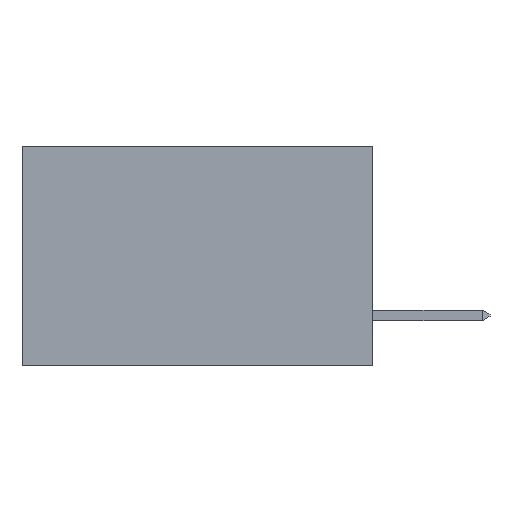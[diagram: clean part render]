
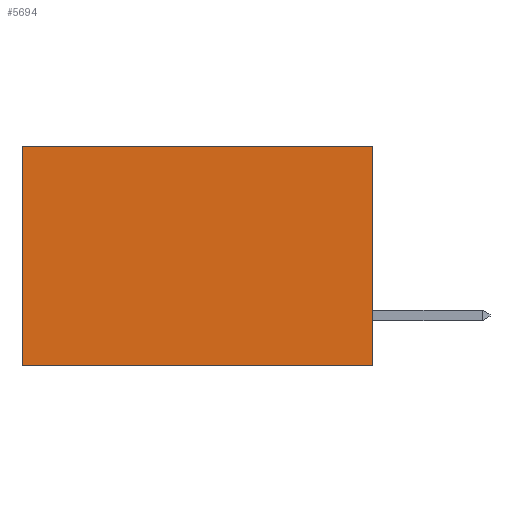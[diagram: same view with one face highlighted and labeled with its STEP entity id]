
A CAD part, left-side view. The second image highlights one B-rep face of the part: STEP entity #5694.
In plain terms, the highlighted planar face has unit normal (-1, 0, 0).
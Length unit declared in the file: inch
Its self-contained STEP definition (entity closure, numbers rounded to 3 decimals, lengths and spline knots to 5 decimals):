
#236 = AXIS2_PLACEMENT_3D ( 'NONE', #5465, #4556, #4618 ) ;
#449 = LINE ( 'NONE', #5411, #7240 ) ;
#672 = VERTEX_POINT ( 'NONE', #8423 ) ;
#1122 = DIRECTION ( 'NONE',  ( 0., 1., 0. ) ) ;
#1736 = EDGE_LOOP ( 'NONE', ( #2048, #1748, #2579, #3522 ) ) ;
#1748 = ORIENTED_EDGE ( 'NONE', *, *, #2026, .F. ) ;
#1870 = LINE ( 'NONE', #3115, #6932 ) ;
#2026 = EDGE_CURVE ( 'NONE', #7557, #6069, #7867, .T. ) ;
#2048 = ORIENTED_EDGE ( 'NONE', *, *, #3025, .T. ) ;
#2579 = ORIENTED_EDGE ( 'NONE', *, *, #5147, .F. ) ;
#2893 = PLANE ( 'NONE',  #236 ) ;
#3025 = EDGE_CURVE ( 'NONE', #672, #6069, #449, .T. ) ;
#3115 = CARTESIAN_POINT ( 'NONE',  ( 0.277, 0., 0. ) ) ;
#3223 = EDGE_CURVE ( 'NONE', #8510, #672, #1870, .T. ) ;
#3522 = ORIENTED_EDGE ( 'NONE', *, *, #3223, .T. ) ;
#4412 = VECTOR ( 'NONE', #7350, 39.37008 ) ;
#4425 = VECTOR ( 'NONE', #6179, 39.37008 ) ;
#4556 = DIRECTION ( 'NONE',  ( 1., 0., 0. ) ) ;
#4618 = DIRECTION ( 'NONE',  ( 0., 0., -1. ) ) ;
#4619 = LINE ( 'NONE', #7349, #4412 ) ;
#4814 = CARTESIAN_POINT ( 'NONE',  ( 0.277, 0., -0.37 ) ) ;
#5106 = FACE_OUTER_BOUND ( 'NONE', #1736, .T. ) ;
#5129 = DIRECTION ( 'NONE',  ( 0., 0., -1. ) ) ;
#5147 = EDGE_CURVE ( 'NONE', #8510, #7557, #4619, .T. ) ;
#5411 = CARTESIAN_POINT ( 'NONE',  ( 0.277, 0.59, -0.37 ) ) ;
#5465 = CARTESIAN_POINT ( 'NONE',  ( 0.277, 0., -0.37 ) ) ;
#5597 = CARTESIAN_POINT ( 'NONE',  ( 0.277, 0., 0. ) ) ;
#5694 = ADVANCED_FACE ( 'NONE', ( #5106 ), #2893, .F. ) ;
#6069 = VERTEX_POINT ( 'NONE', #8297 ) ;
#6074 = CARTESIAN_POINT ( 'NONE',  ( 0.277, 0., -0.37 ) ) ;
#6179 = DIRECTION ( 'NONE',  ( 0., 1., 0. ) ) ;
#6932 = VECTOR ( 'NONE', #1122, 39.37008 ) ;
#7240 = VECTOR ( 'NONE', #5129, 39.37008 ) ;
#7349 = CARTESIAN_POINT ( 'NONE',  ( 0.277, 0., -0.37 ) ) ;
#7350 = DIRECTION ( 'NONE',  ( 0., 0., -1. ) ) ;
#7557 = VERTEX_POINT ( 'NONE', #4814 ) ;
#7867 = LINE ( 'NONE', #6074, #4425 ) ;
#8297 = CARTESIAN_POINT ( 'NONE',  ( 0.277, 0.59, -0.37 ) ) ;
#8423 = CARTESIAN_POINT ( 'NONE',  ( 0.277, 0.59, 0. ) ) ;
#8510 = VERTEX_POINT ( 'NONE', #5597 ) ;
